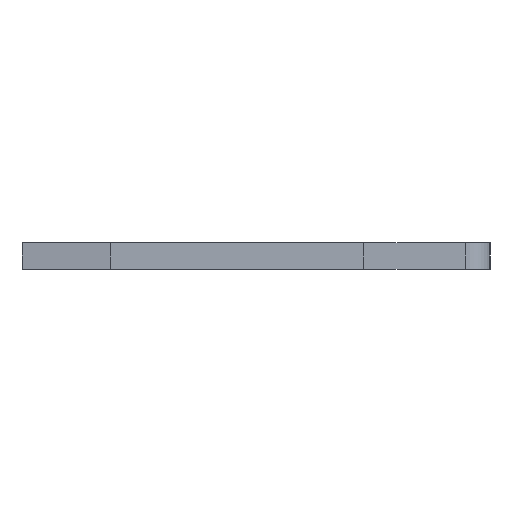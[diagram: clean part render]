
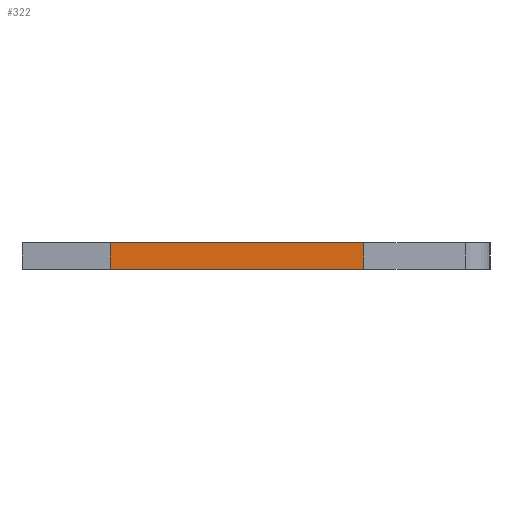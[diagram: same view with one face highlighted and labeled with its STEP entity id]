
A CAD part, left-side view. The second image highlights one B-rep face of the part: STEP entity #322.
In plain terms, the highlighted face is planar.
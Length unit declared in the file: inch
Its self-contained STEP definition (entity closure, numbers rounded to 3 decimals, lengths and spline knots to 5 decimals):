
#15 = ORIENTED_EDGE ( 'NONE', *, *, #787, .F. ) ;
#47 = LINE ( 'NONE', #91, #152 ) ;
#66 = EDGE_CURVE ( 'NONE', #99, #966, #844, .T. ) ;
#74 = DIRECTION ( 'NONE',  ( -1., 0., 0. ) ) ;
#91 = CARTESIAN_POINT ( 'NONE',  ( 0.013, -0.099, -0.0575 ) ) ;
#99 = VERTEX_POINT ( 'NONE', #157 ) ;
#103 = CARTESIAN_POINT ( 'NONE',  ( 0.013, 0.146, -0.0575 ) ) ;
#114 = DIRECTION ( 'NONE',  ( 0., 0., 1. ) ) ;
#152 = VECTOR ( 'NONE', #74, 39.37008 ) ;
#157 = CARTESIAN_POINT ( 'NONE',  ( 0.013, -0.099, -0.0575 ) ) ;
#225 = EDGE_LOOP ( 'NONE', ( #909, #15, #1039, #1223 ) ) ;
#263 = DIRECTION ( 'NONE',  ( 0., 1., 0. ) ) ;
#264 = EDGE_CURVE ( 'NONE', #99, #371, #47, .T. ) ;
#273 = FACE_OUTER_BOUND ( 'NONE', #225, .T. ) ;
#322 = ADVANCED_FACE ( 'NONE', ( #273 ), #967, .F. ) ;
#344 = DIRECTION ( 'NONE',  ( 0., 1., 0. ) ) ;
#371 = VERTEX_POINT ( 'NONE', #419 ) ;
#377 = AXIS2_PLACEMENT_3D ( 'NONE', #103, #114, #1206 ) ;
#419 = CARTESIAN_POINT ( 'NONE',  ( -0.013, -0.099, -0.0575 ) ) ;
#473 = CARTESIAN_POINT ( 'NONE',  ( 0.013, 0.146, -0.0575 ) ) ;
#622 = CARTESIAN_POINT ( 'NONE',  ( -0.013, 0.146, -0.0575 ) ) ;
#730 = VERTEX_POINT ( 'NONE', #622 ) ;
#749 = VECTOR ( 'NONE', #263, 39.37008 ) ;
#760 = CARTESIAN_POINT ( 'NONE',  ( 0.013, 0.146, -0.0575 ) ) ;
#787 = EDGE_CURVE ( 'NONE', #966, #730, #1247, .T. ) ;
#794 = VECTOR ( 'NONE', #985, 39.37008 ) ;
#844 = LINE ( 'NONE', #473, #749 ) ;
#909 = ORIENTED_EDGE ( 'NONE', *, *, #1218, .T. ) ;
#957 = VECTOR ( 'NONE', #344, 39.37008 ) ;
#966 = VERTEX_POINT ( 'NONE', #1337 ) ;
#967 = PLANE ( 'NONE',  #377 ) ;
#985 = DIRECTION ( 'NONE',  ( -1., 0., 0. ) ) ;
#1039 = ORIENTED_EDGE ( 'NONE', *, *, #66, .F. ) ;
#1042 = CARTESIAN_POINT ( 'NONE',  ( -0.013, 0.146, -0.0575 ) ) ;
#1206 = DIRECTION ( 'NONE',  ( 1., 0., 0. ) ) ;
#1213 = LINE ( 'NONE', #1042, #957 ) ;
#1218 = EDGE_CURVE ( 'NONE', #371, #730, #1213, .T. ) ;
#1223 = ORIENTED_EDGE ( 'NONE', *, *, #264, .T. ) ;
#1247 = LINE ( 'NONE', #760, #794 ) ;
#1337 = CARTESIAN_POINT ( 'NONE',  ( 0.013, 0.146, -0.0575 ) ) ;
